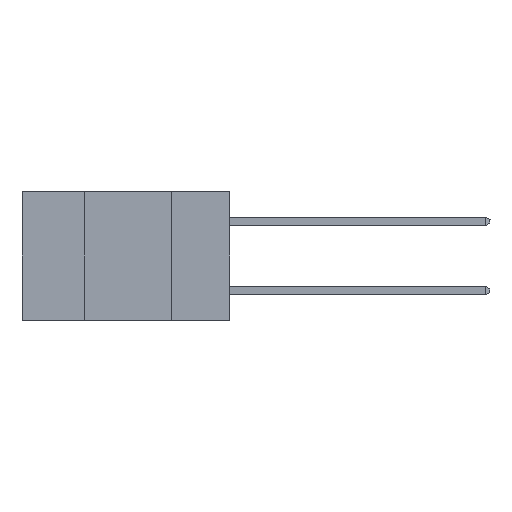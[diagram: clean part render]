
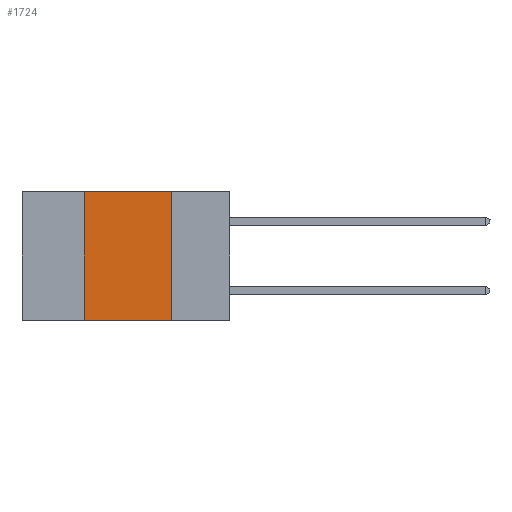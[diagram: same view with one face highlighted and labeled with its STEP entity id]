
A CAD part, left-side view. The second image highlights one B-rep face of the part: STEP entity #1724.
In plain terms, the highlighted planar face has unit normal (-1, 0, 0).
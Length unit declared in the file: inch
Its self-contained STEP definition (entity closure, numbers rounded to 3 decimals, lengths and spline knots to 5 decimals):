
#490 = DIRECTION ( 'NONE',  ( 0., -1., 0. ) ) ;
#561 = ORIENTED_EDGE ( 'NONE', *, *, #6265, .F. ) ;
#797 = VERTEX_POINT ( 'NONE', #2825 ) ;
#1724 = ADVANCED_FACE ( 'NONE', ( #12428 ), #12611, .F. ) ;
#2787 = VECTOR ( 'NONE', #490, 39.37008 ) ;
#2825 = CARTESIAN_POINT ( 'NONE',  ( 0., 0.17, 0. ) ) ;
#3704 = DIRECTION ( 'NONE',  ( 1., 0., 0. ) ) ;
#4670 = EDGE_CURVE ( 'NONE', #797, #14448, #16407, .T. ) ;
#5719 = VERTEX_POINT ( 'NONE', #18072 ) ;
#6265 = EDGE_CURVE ( 'NONE', #5719, #16369, #16650, .T. ) ;
#6481 = LINE ( 'NONE', #17984, #2787 ) ;
#6983 = CARTESIAN_POINT ( 'NONE',  ( 0., 0.6, 0. ) ) ;
#7086 = VECTOR ( 'NONE', #18177, 39.37008 ) ;
#10708 = EDGE_CURVE ( 'NONE', #5719, #14448, #12328, .T. ) ;
#11350 = VECTOR ( 'NONE', #15052, 39.37008 ) ;
#12060 = DIRECTION ( 'NONE',  ( 0., -1., 0. ) ) ;
#12089 = VECTOR ( 'NONE', #12060, 39.37008 ) ;
#12328 = LINE ( 'NONE', #18195, #12089 ) ;
#12428 = FACE_OUTER_BOUND ( 'NONE', #13338, .T. ) ;
#12611 = PLANE ( 'NONE',  #13751 ) ;
#13338 = EDGE_LOOP ( 'NONE', ( #14331, #14069, #561, #13551 ) ) ;
#13551 = ORIENTED_EDGE ( 'NONE', *, *, #10708, .T. ) ;
#13751 = AXIS2_PLACEMENT_3D ( 'NONE', #6983, #3704, #15069 ) ;
#14069 = ORIENTED_EDGE ( 'NONE', *, *, #16426, .F. ) ;
#14331 = ORIENTED_EDGE ( 'NONE', *, *, #4670, .F. ) ;
#14448 = VERTEX_POINT ( 'NONE', #18720 ) ;
#15052 = DIRECTION ( 'NONE',  ( 0., 0., -1. ) ) ;
#15069 = DIRECTION ( 'NONE',  ( 0., 0., -1. ) ) ;
#16207 = CARTESIAN_POINT ( 'NONE',  ( 0., 0.17, -0.37 ) ) ;
#16351 = CARTESIAN_POINT ( 'NONE',  ( 0., 0.42, 0. ) ) ;
#16369 = VERTEX_POINT ( 'NONE', #16351 ) ;
#16407 = LINE ( 'NONE', #16207, #11350 ) ;
#16426 = EDGE_CURVE ( 'NONE', #16369, #797, #6481, .T. ) ;
#16650 = LINE ( 'NONE', #18272, #7086 ) ;
#17984 = CARTESIAN_POINT ( 'NONE',  ( 0., 0.6, 0. ) ) ;
#18072 = CARTESIAN_POINT ( 'NONE',  ( 0., 0.42, -0.37 ) ) ;
#18177 = DIRECTION ( 'NONE',  ( 0., 0., 1. ) ) ;
#18195 = CARTESIAN_POINT ( 'NONE',  ( 0., 0.6, -0.37 ) ) ;
#18272 = CARTESIAN_POINT ( 'NONE',  ( 0., 0.42, -0.37 ) ) ;
#18720 = CARTESIAN_POINT ( 'NONE',  ( 0., 0.17, -0.37 ) ) ;
